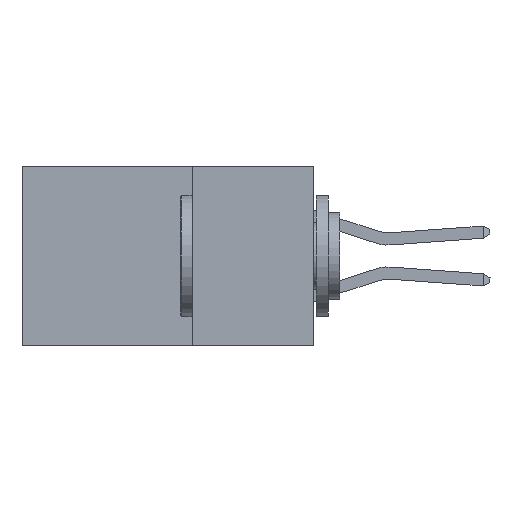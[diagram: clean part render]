
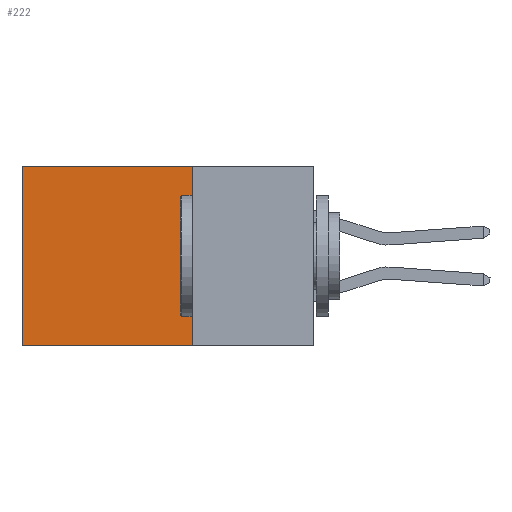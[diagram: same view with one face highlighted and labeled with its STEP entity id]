
A CAD part, left-side view. The second image highlights one B-rep face of the part: STEP entity #222.
In plain terms, the highlighted planar face has unit normal (-1, 0, 0).
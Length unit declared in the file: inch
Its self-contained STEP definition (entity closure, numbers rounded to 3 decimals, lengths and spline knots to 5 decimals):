
#222 = ADVANCED_FACE ( 'NONE', ( #14788 ), #8357, .F. ) ;
#262 = LINE ( 'NONE', #1308, #14765 ) ;
#632 = EDGE_CURVE ( 'NONE', #5824, #6540, #9861, .T. ) ;
#1308 = CARTESIAN_POINT ( 'NONE',  ( 0.2875, 0.25, 0. ) ) ;
#1427 = VECTOR ( 'NONE', #10222, 39.37008 ) ;
#1937 = EDGE_LOOP ( 'NONE', ( #3914, #7287, #10282, #10993 ) ) ;
#2636 = VERTEX_POINT ( 'NONE', #10581 ) ;
#3123 = CARTESIAN_POINT ( 'NONE',  ( 0.2875, 0.25, -0.37 ) ) ;
#3269 = DIRECTION ( 'NONE',  ( 0., 0., -1. ) ) ;
#3570 = CARTESIAN_POINT ( 'NONE',  ( 0.2875, 0.25, 0. ) ) ;
#3905 = DIRECTION ( 'NONE',  ( 0., 0., -1. ) ) ;
#3914 = ORIENTED_EDGE ( 'NONE', *, *, #11859, .T. ) ;
#3925 = DIRECTION ( 'NONE',  ( 1., 0., 0. ) ) ;
#3930 = DIRECTION ( 'NONE',  ( 0., 1., 0. ) ) ;
#4883 = CARTESIAN_POINT ( 'NONE',  ( 0.2875, 0.25, 0. ) ) ;
#5647 = EDGE_CURVE ( 'NONE', #5824, #2636, #262, .T. ) ;
#5824 = VERTEX_POINT ( 'NONE', #10886 ) ;
#5976 = VECTOR ( 'NONE', #3930, 39.37008 ) ;
#6516 = VECTOR ( 'NONE', #3269, 39.37008 ) ;
#6540 = VERTEX_POINT ( 'NONE', #3123 ) ;
#7287 = ORIENTED_EDGE ( 'NONE', *, *, #10707, .F. ) ;
#8357 = PLANE ( 'NONE',  #9848 ) ;
#9113 = CARTESIAN_POINT ( 'NONE',  ( 0.2875, 0.6, 0. ) ) ;
#9355 = VERTEX_POINT ( 'NONE', #9678 ) ;
#9678 = CARTESIAN_POINT ( 'NONE',  ( 0.2875, 0.6, -0.37 ) ) ;
#9848 = AXIS2_PLACEMENT_3D ( 'NONE', #3570, #3925, #3905 ) ;
#9861 = LINE ( 'NONE', #4883, #6516 ) ;
#10040 = LINE ( 'NONE', #10710, #5976 ) ;
#10222 = DIRECTION ( 'NONE',  ( 0., 0., -1. ) ) ;
#10282 = ORIENTED_EDGE ( 'NONE', *, *, #632, .F. ) ;
#10581 = CARTESIAN_POINT ( 'NONE',  ( 0.2875, 0.6, 0. ) ) ;
#10707 = EDGE_CURVE ( 'NONE', #6540, #9355, #10040, .T. ) ;
#10710 = CARTESIAN_POINT ( 'NONE',  ( 0.2875, 0.25, -0.37 ) ) ;
#10886 = CARTESIAN_POINT ( 'NONE',  ( 0.2875, 0.25, 0. ) ) ;
#10993 = ORIENTED_EDGE ( 'NONE', *, *, #5647, .T. ) ;
#11016 = LINE ( 'NONE', #9113, #1427 ) ;
#11682 = DIRECTION ( 'NONE',  ( 0., 1., 0. ) ) ;
#11859 = EDGE_CURVE ( 'NONE', #2636, #9355, #11016, .T. ) ;
#14765 = VECTOR ( 'NONE', #11682, 39.37008 ) ;
#14788 = FACE_OUTER_BOUND ( 'NONE', #1937, .T. ) ;
